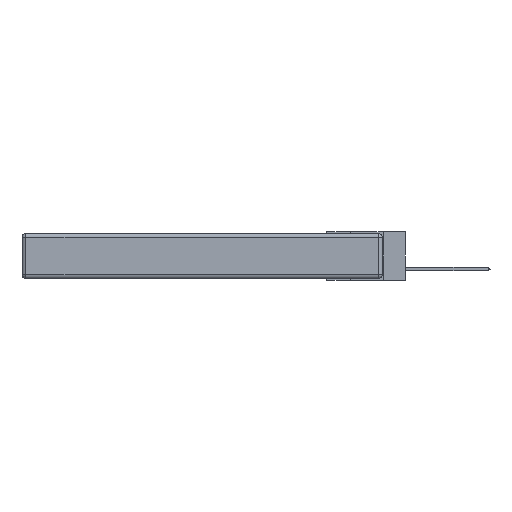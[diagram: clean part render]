
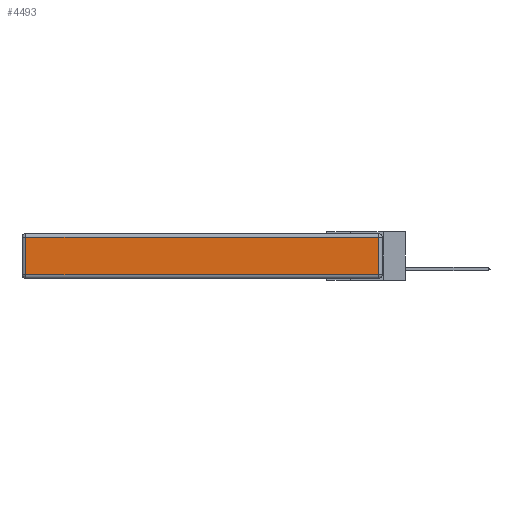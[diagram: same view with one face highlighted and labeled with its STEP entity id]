
A CAD part, left-side view. The second image highlights one B-rep face of the part: STEP entity #4493.
In plain terms, the highlighted planar face has unit normal (-1, 0, 0).
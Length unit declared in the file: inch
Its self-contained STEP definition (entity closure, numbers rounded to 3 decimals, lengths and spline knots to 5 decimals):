
#769 = CARTESIAN_POINT ( 'NONE',  ( 0., 2.72, -0.03 ) ) ;
#3105 = LINE ( 'NONE', #4950, #26534 ) ;
#3253 = ORIENTED_EDGE ( 'NONE', *, *, #13866, .T. ) ;
#4134 = LINE ( 'NONE', #26508, #9881 ) ;
#4332 = ORIENTED_EDGE ( 'NONE', *, *, #21828, .T. ) ;
#4493 = ADVANCED_FACE ( 'NONE', ( #27227 ), #11096, .T. ) ;
#4628 = CARTESIAN_POINT ( 'NONE',  ( 0., 0.03, -0.03 ) ) ;
#4874 = EDGE_CURVE ( 'NONE', #18364, #11370, #3105, .T. ) ;
#4950 = CARTESIAN_POINT ( 'NONE',  ( 0., 2.72, -0.343 ) ) ;
#6355 = CARTESIAN_POINT ( 'NONE',  ( 0., 0., -0.343 ) ) ;
#7120 = EDGE_CURVE ( 'NONE', #7461, #17992, #27869, .T. ) ;
#7461 = VERTEX_POINT ( 'NONE', #14510 ) ;
#9396 = DIRECTION ( 'NONE',  ( 0., 0., -1. ) ) ;
#9715 = CARTESIAN_POINT ( 'NONE',  ( 0., 2.72, -0.313 ) ) ;
#9881 = VECTOR ( 'NONE', #28816, 39.37008 ) ;
#9961 = DIRECTION ( 'NONE',  ( 0., 0., 1. ) ) ;
#10036 = DIRECTION ( 'NONE',  ( 0., 0., 1. ) ) ;
#11096 = PLANE ( 'NONE',  #23703 ) ;
#11370 = VERTEX_POINT ( 'NONE', #9715 ) ;
#12934 = CARTESIAN_POINT ( 'NONE',  ( 0., 2.75, -0.03 ) ) ;
#13459 = VECTOR ( 'NONE', #10036, 39.37008 ) ;
#13722 = ORIENTED_EDGE ( 'NONE', *, *, #7120, .T. ) ;
#13866 = EDGE_CURVE ( 'NONE', #17992, #18364, #21967, .T. ) ;
#14510 = CARTESIAN_POINT ( 'NONE',  ( 0., 0.03, -0.313 ) ) ;
#17992 = VERTEX_POINT ( 'NONE', #4628 ) ;
#18364 = VERTEX_POINT ( 'NONE', #769 ) ;
#20162 = ORIENTED_EDGE ( 'NONE', *, *, #4874, .T. ) ;
#21121 = DIRECTION ( 'NONE',  ( -1., 0., 0. ) ) ;
#21828 = EDGE_CURVE ( 'NONE', #11370, #7461, #4134, .T. ) ;
#21967 = LINE ( 'NONE', #12934, #23403 ) ;
#23403 = VECTOR ( 'NONE', #24520, 39.37008 ) ;
#23703 = AXIS2_PLACEMENT_3D ( 'NONE', #6355, #21121, #9961 ) ;
#23900 = EDGE_LOOP ( 'NONE', ( #4332, #13722, #3253, #20162 ) ) ;
#24520 = DIRECTION ( 'NONE',  ( 0., 1., 0. ) ) ;
#26114 = CARTESIAN_POINT ( 'NONE',  ( 0., 0.03, -0.343 ) ) ;
#26508 = CARTESIAN_POINT ( 'NONE',  ( 0., 0., -0.313 ) ) ;
#26534 = VECTOR ( 'NONE', #9396, 39.37008 ) ;
#27227 = FACE_OUTER_BOUND ( 'NONE', #23900, .T. ) ;
#27869 = LINE ( 'NONE', #26114, #13459 ) ;
#28816 = DIRECTION ( 'NONE',  ( 0., -1., 0. ) ) ;
